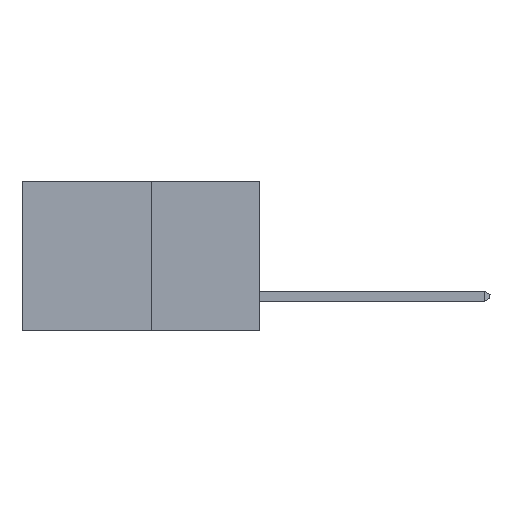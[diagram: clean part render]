
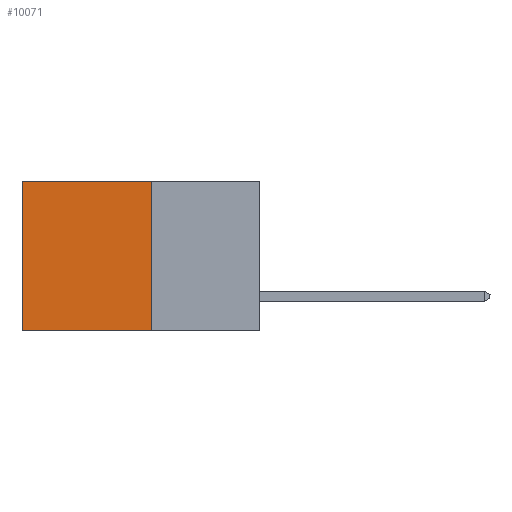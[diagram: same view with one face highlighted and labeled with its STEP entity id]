
A CAD part, left-side view. The second image highlights one B-rep face of the part: STEP entity #10071.
In plain terms, the highlighted planar face has unit normal (-1, 0, 0).
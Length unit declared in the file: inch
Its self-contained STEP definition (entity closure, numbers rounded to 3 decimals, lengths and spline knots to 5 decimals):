
#25 = CARTESIAN_POINT ( 'NONE',  ( 0.277, 0.27, 0. ) ) ;
#91 = DIRECTION ( 'NONE',  ( 1., 0., 0. ) ) ;
#860 = ORIENTED_EDGE ( 'NONE', *, *, #2140, .F. ) ;
#2140 = EDGE_CURVE ( 'NONE', #5870, #6414, #14545, .T. ) ;
#2257 = EDGE_CURVE ( 'NONE', #6414, #8387, #13141, .T. ) ;
#2422 = FACE_OUTER_BOUND ( 'NONE', #4866, .T. ) ;
#3083 = LINE ( 'NONE', #5404, #13069 ) ;
#3552 = VECTOR ( 'NONE', #15331, 39.37008 ) ;
#3828 = PLANE ( 'NONE',  #14032 ) ;
#4866 = EDGE_LOOP ( 'NONE', ( #7201, #11436, #860, #5924 ) ) ;
#5084 = VECTOR ( 'NONE', #11015, 39.37008 ) ;
#5228 = EDGE_CURVE ( 'NONE', #5870, #13317, #7931, .T. ) ;
#5404 = CARTESIAN_POINT ( 'NONE',  ( 0.277, 0.59, -0.37 ) ) ;
#5870 = VERTEX_POINT ( 'NONE', #25 ) ;
#5924 = ORIENTED_EDGE ( 'NONE', *, *, #5228, .T. ) ;
#6414 = VERTEX_POINT ( 'NONE', #7383 ) ;
#6674 = EDGE_CURVE ( 'NONE', #13317, #8387, #3083, .T. ) ;
#7201 = ORIENTED_EDGE ( 'NONE', *, *, #6674, .T. ) ;
#7383 = CARTESIAN_POINT ( 'NONE',  ( 0.277, 0.27, -0.37 ) ) ;
#7527 = CARTESIAN_POINT ( 'NONE',  ( 0.277, 0.27, -0.37 ) ) ;
#7931 = LINE ( 'NONE', #13668, #13809 ) ;
#8387 = VERTEX_POINT ( 'NONE', #11989 ) ;
#8720 = DIRECTION ( 'NONE',  ( 0., 0., -1. ) ) ;
#10071 = ADVANCED_FACE ( 'NONE', ( #2422 ), #3828, .F. ) ;
#10208 = DIRECTION ( 'NONE',  ( 0., 0., -1. ) ) ;
#11015 = DIRECTION ( 'NONE',  ( 0., 0., -1. ) ) ;
#11436 = ORIENTED_EDGE ( 'NONE', *, *, #2257, .F. ) ;
#11989 = CARTESIAN_POINT ( 'NONE',  ( 0.277, 0.59, -0.37 ) ) ;
#12053 = CARTESIAN_POINT ( 'NONE',  ( 0.277, 0.59, 0. ) ) ;
#13069 = VECTOR ( 'NONE', #10208, 39.37008 ) ;
#13141 = LINE ( 'NONE', #15387, #3552 ) ;
#13207 = CARTESIAN_POINT ( 'NONE',  ( 0.277, 0.27, -0.37 ) ) ;
#13317 = VERTEX_POINT ( 'NONE', #12053 ) ;
#13529 = DIRECTION ( 'NONE',  ( 0., 1., 0. ) ) ;
#13668 = CARTESIAN_POINT ( 'NONE',  ( 0.277, 0.27, 0. ) ) ;
#13809 = VECTOR ( 'NONE', #13529, 39.37008 ) ;
#14032 = AXIS2_PLACEMENT_3D ( 'NONE', #7527, #91, #8720 ) ;
#14545 = LINE ( 'NONE', #13207, #5084 ) ;
#15331 = DIRECTION ( 'NONE',  ( 0., 1., 0. ) ) ;
#15387 = CARTESIAN_POINT ( 'NONE',  ( 0.277, 0.27, -0.37 ) ) ;
